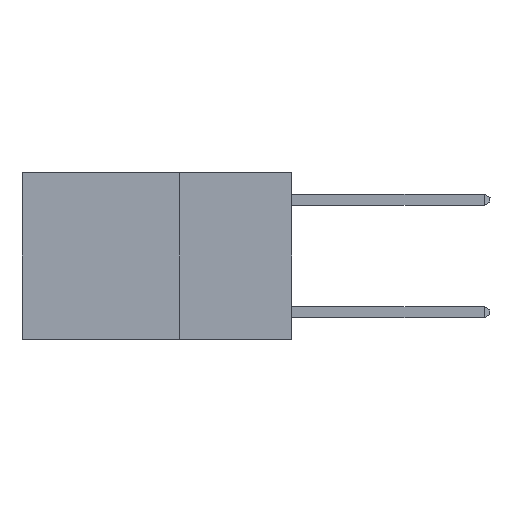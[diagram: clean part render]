
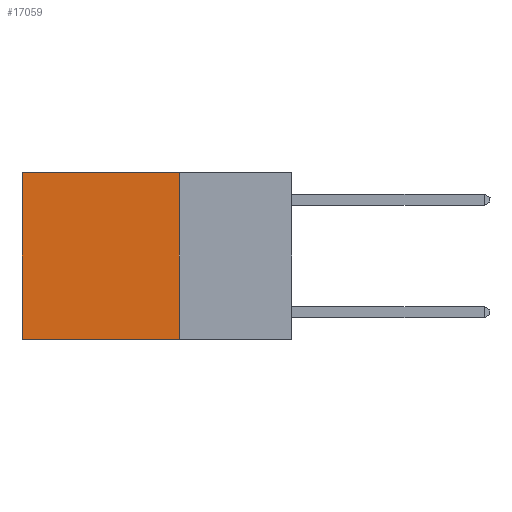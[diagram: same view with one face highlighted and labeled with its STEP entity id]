
A CAD part, left-side view. The second image highlights one B-rep face of the part: STEP entity #17059.
In plain terms, the highlighted planar face has unit normal (-1, 0, 0).
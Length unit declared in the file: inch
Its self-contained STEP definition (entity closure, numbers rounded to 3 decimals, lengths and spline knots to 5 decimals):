
#138 = CARTESIAN_POINT ( 'NONE',  ( 0.2625, 0.25, -0.37 ) ) ;
#374 = VECTOR ( 'NONE', #5795, 39.37008 ) ;
#1681 = VECTOR ( 'NONE', #19812, 39.37008 ) ;
#2164 = LINE ( 'NONE', #9029, #18132 ) ;
#3552 = CARTESIAN_POINT ( 'NONE',  ( 0.2625, 0.25, 0. ) ) ;
#4337 = CARTESIAN_POINT ( 'NONE',  ( 0.2625, 0.6, -0.37 ) ) ;
#4407 = AXIS2_PLACEMENT_3D ( 'NONE', #9429, #7824, #16454 ) ;
#4698 = EDGE_CURVE ( 'NONE', #13800, #22148, #17809, .T. ) ;
#5246 = VERTEX_POINT ( 'NONE', #6378 ) ;
#5795 = DIRECTION ( 'NONE',  ( 0., 0., -1. ) ) ;
#6378 = CARTESIAN_POINT ( 'NONE',  ( 0.2625, 0.6, 0. ) ) ;
#6927 = CARTESIAN_POINT ( 'NONE',  ( 0.2625, 0.25, 0. ) ) ;
#7824 = DIRECTION ( 'NONE',  ( 1., 0., 0. ) ) ;
#9029 = CARTESIAN_POINT ( 'NONE',  ( 0.2625, 0.25, -0.37 ) ) ;
#9315 = PLANE ( 'NONE',  #4407 ) ;
#9429 = CARTESIAN_POINT ( 'NONE',  ( 0.2625, 0.25, 0. ) ) ;
#11278 = FACE_OUTER_BOUND ( 'NONE', #13060, .T. ) ;
#13060 = EDGE_LOOP ( 'NONE', ( #17691, #21660, #15314, #13378 ) ) ;
#13248 = VERTEX_POINT ( 'NONE', #4337 ) ;
#13378 = ORIENTED_EDGE ( 'NONE', *, *, #15361, .T. ) ;
#13475 = EDGE_CURVE ( 'NONE', #22148, #13248, #2164, .T. ) ;
#13800 = VERTEX_POINT ( 'NONE', #6927 ) ;
#14973 = VECTOR ( 'NONE', #21364, 39.37008 ) ;
#15314 = ORIENTED_EDGE ( 'NONE', *, *, #4698, .F. ) ;
#15361 = EDGE_CURVE ( 'NONE', #13800, #5246, #21442, .T. ) ;
#16454 = DIRECTION ( 'NONE',  ( 0., 0., -1. ) ) ;
#16712 = EDGE_CURVE ( 'NONE', #5246, #13248, #19935, .T. ) ;
#17059 = ADVANCED_FACE ( 'NONE', ( #11278 ), #9315, .F. ) ;
#17691 = ORIENTED_EDGE ( 'NONE', *, *, #16712, .T. ) ;
#17809 = LINE ( 'NONE', #3552, #14973 ) ;
#18004 = DIRECTION ( 'NONE',  ( 0., 1., 0. ) ) ;
#18132 = VECTOR ( 'NONE', #18004, 39.37008 ) ;
#19812 = DIRECTION ( 'NONE',  ( 0., 1., 0. ) ) ;
#19817 = CARTESIAN_POINT ( 'NONE',  ( 0.2625, 0.6, 0. ) ) ;
#19935 = LINE ( 'NONE', #19817, #374 ) ;
#21364 = DIRECTION ( 'NONE',  ( 0., 0., -1. ) ) ;
#21442 = LINE ( 'NONE', #21668, #1681 ) ;
#21660 = ORIENTED_EDGE ( 'NONE', *, *, #13475, .F. ) ;
#21668 = CARTESIAN_POINT ( 'NONE',  ( 0.2625, 0.25, 0. ) ) ;
#22148 = VERTEX_POINT ( 'NONE', #138 ) ;
